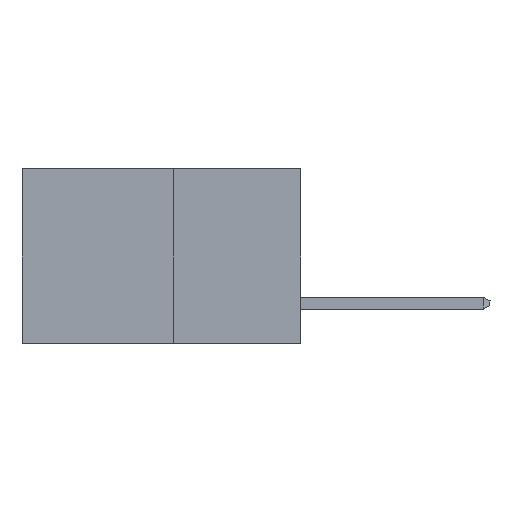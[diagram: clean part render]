
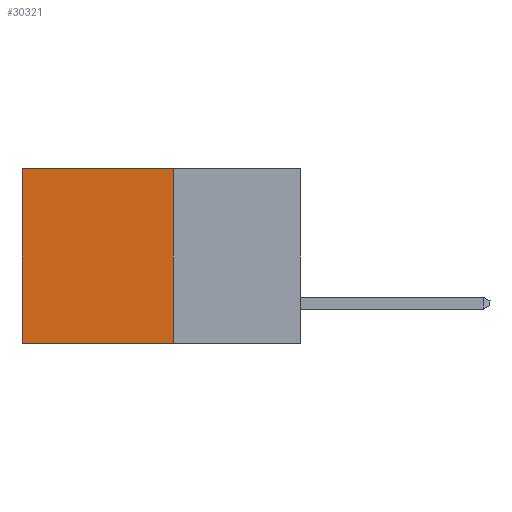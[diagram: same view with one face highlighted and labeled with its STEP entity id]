
A CAD part, left-side view. The second image highlights one B-rep face of the part: STEP entity #30321.
In plain terms, the highlighted planar face has unit normal (-1, 0, 0).
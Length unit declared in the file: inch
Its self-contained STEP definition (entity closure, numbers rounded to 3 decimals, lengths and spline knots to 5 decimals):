
#1117 = DIRECTION ( 'NONE',  ( 0., 0., -1. ) ) ;
#1301 = LINE ( 'NONE', #3579, #20374 ) ;
#2278 = LINE ( 'NONE', #3205, #8932 ) ;
#2518 = LINE ( 'NONE', #18514, #22372 ) ;
#3205 = CARTESIAN_POINT ( 'NONE',  ( 0.277, 0.27, 0. ) ) ;
#3579 = CARTESIAN_POINT ( 'NONE',  ( 0.277, 0.27, -0.37 ) ) ;
#5744 = DIRECTION ( 'NONE',  ( 0., 1., 0. ) ) ;
#6273 = CARTESIAN_POINT ( 'NONE',  ( 0.277, 0.59, -0.37 ) ) ;
#6858 = DIRECTION ( 'NONE',  ( 0., 0., -1. ) ) ;
#8407 = CARTESIAN_POINT ( 'NONE',  ( 0.277, 0.59, 0. ) ) ;
#8836 = VECTOR ( 'NONE', #6858, 39.37008 ) ;
#8932 = VECTOR ( 'NONE', #5744, 39.37008 ) ;
#12532 = DIRECTION ( 'NONE',  ( 1., 0., 0. ) ) ;
#12996 = FACE_OUTER_BOUND ( 'NONE', #29913, .T. ) ;
#14886 = ORIENTED_EDGE ( 'NONE', *, *, #16224, .T. ) ;
#15310 = CARTESIAN_POINT ( 'NONE',  ( 0.277, 0.27, 0. ) ) ;
#16224 = EDGE_CURVE ( 'NONE', #30584, #16741, #28706, .T. ) ;
#16741 = VERTEX_POINT ( 'NONE', #6273 ) ;
#17280 = EDGE_CURVE ( 'NONE', #30442, #23268, #2518, .T. ) ;
#17954 = EDGE_CURVE ( 'NONE', #23268, #16741, #1301, .T. ) ;
#18514 = CARTESIAN_POINT ( 'NONE',  ( 0.277, 0.27, -0.37 ) ) ;
#20262 = EDGE_CURVE ( 'NONE', #30442, #30584, #2278, .T. ) ;
#20374 = VECTOR ( 'NONE', #26035, 39.37008 ) ;
#21353 = AXIS2_PLACEMENT_3D ( 'NONE', #29849, #12532, #29948 ) ;
#22372 = VECTOR ( 'NONE', #1117, 39.37008 ) ;
#23268 = VERTEX_POINT ( 'NONE', #26699 ) ;
#24782 = ORIENTED_EDGE ( 'NONE', *, *, #17954, .F. ) ;
#25609 = ORIENTED_EDGE ( 'NONE', *, *, #20262, .T. ) ;
#26035 = DIRECTION ( 'NONE',  ( 0., 1., 0. ) ) ;
#26699 = CARTESIAN_POINT ( 'NONE',  ( 0.277, 0.27, -0.37 ) ) ;
#26774 = CARTESIAN_POINT ( 'NONE',  ( 0.277, 0.59, -0.37 ) ) ;
#26977 = ORIENTED_EDGE ( 'NONE', *, *, #17280, .F. ) ;
#27456 = PLANE ( 'NONE',  #21353 ) ;
#28706 = LINE ( 'NONE', #26774, #8836 ) ;
#29849 = CARTESIAN_POINT ( 'NONE',  ( 0.277, 0.27, -0.37 ) ) ;
#29913 = EDGE_LOOP ( 'NONE', ( #14886, #24782, #26977, #25609 ) ) ;
#29948 = DIRECTION ( 'NONE',  ( 0., 0., -1. ) ) ;
#30321 = ADVANCED_FACE ( 'NONE', ( #12996 ), #27456, .F. ) ;
#30442 = VERTEX_POINT ( 'NONE', #15310 ) ;
#30584 = VERTEX_POINT ( 'NONE', #8407 ) ;
